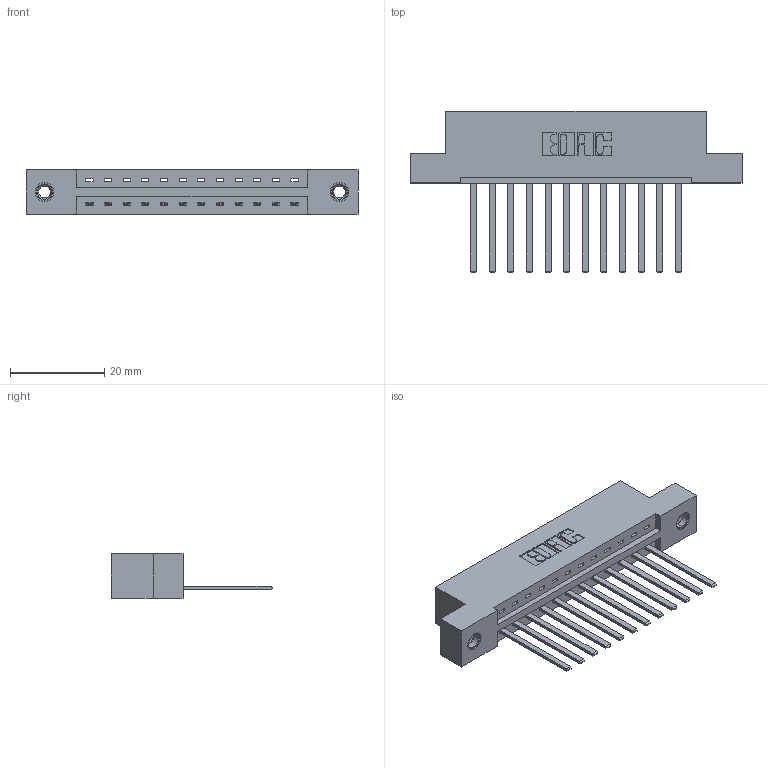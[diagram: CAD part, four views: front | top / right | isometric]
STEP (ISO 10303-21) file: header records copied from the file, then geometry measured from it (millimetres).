
FILE_DESCRIPTION (( 'STEP AP203' ), '1' );
FILE_NAME ('337-012-544-107.STEP', '2019-09-28T00:50:31', ( '' ), ( '' ), 'SwSTEP 2.0', 'SolidWorks 2016', '' );
FILE_SCHEMA (( 'CONFIG_CONTROL_DESIGN' ));
Length unit declared in the file: inch
Products named in the file (4): 337-012-544-107; 345-250-001_345-250-005-103; 345-292-001_345-293-144; 337 Part_Flush Mounting Lugs - 0.156 Dia-TI
Assembly tree (15 placements, depth 2):
  337-012-544-107
    337 Part_Flush Mounting Lugs - 0.156 Dia-TI
    345-292-001_345-293-144  x12
    345-250-001_345-250-005-103  x2
Bounding box: 70.56 x 34.3 x 9.4 mm (x, y, z)
Volume: 7083.7 mm3; surface area: 7651.7 mm2
Topology: 15 solids, 15 shells, 846 faces, 2487 edges, 1634 vertices
Faces by surface type: plane 606, cylinder 224, cone 12, torus 4
Entity records: 13802 total; most frequent: CARTESIAN_POINT 2381, ORIENTED_EDGE 2322, DIRECTION 2095, EDGE_CURVE 1161, VECTOR 1017, LINE 1017, VERTEX_POINT 768, AXIS2_PLACEMENT_3D 539
